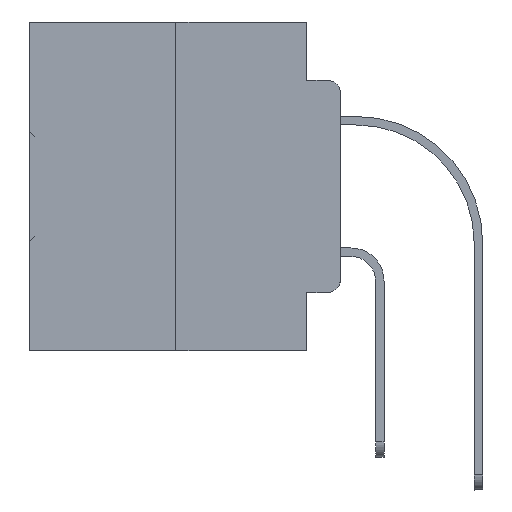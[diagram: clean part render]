
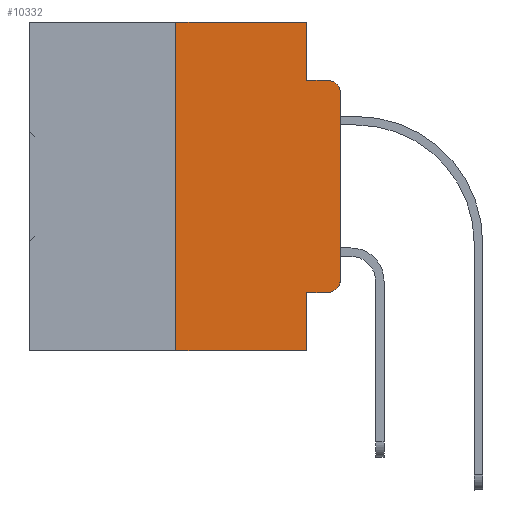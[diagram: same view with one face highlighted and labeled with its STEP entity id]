
A CAD part, left-side view. The second image highlights one B-rep face of the part: STEP entity #10332.
In plain terms, the highlighted planar face has unit normal (-1, 0, 0).
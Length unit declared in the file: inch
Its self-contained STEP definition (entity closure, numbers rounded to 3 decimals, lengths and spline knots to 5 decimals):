
#187 = ORIENTED_EDGE ( 'NONE', *, *, #8697, .T. ) ;
#193 = ORIENTED_EDGE ( 'NONE', *, *, #16590, .F. ) ;
#374 = CARTESIAN_POINT ( 'NONE',  ( 0., 0.051, 0. ) ) ;
#519 = EDGE_CURVE ( 'NONE', #16390, #2244, #39114, .T. ) ;
#630 = CARTESIAN_POINT ( 'NONE',  ( 0., 0.051, 0. ) ) ;
#1103 = ORIENTED_EDGE ( 'NONE', *, *, #519, .T. ) ;
#1309 = EDGE_LOOP ( 'NONE', ( #1103, #26729, #22844, #6492, #193, #5804, #22994, #35599, #187, #27487 ) ) ;
#1374 = DIRECTION ( 'NONE',  ( -1., 0., 0. ) ) ;
#1919 = CARTESIAN_POINT ( 'NONE',  ( 0., 0.051, 0. ) ) ;
#2244 = VERTEX_POINT ( 'NONE', #14629 ) ;
#3180 = VECTOR ( 'NONE', #23820, 39.37008 ) ;
#3497 = EDGE_CURVE ( 'NONE', #2244, #32192, #19511, .T. ) ;
#3555 = DIRECTION ( 'NONE',  ( 0., 0., -1. ) ) ;
#3801 = CARTESIAN_POINT ( 'NONE',  ( 0., 0.051, -0.0885 ) ) ;
#3880 = CARTESIAN_POINT ( 'NONE',  ( 0., 0.051, -0.4115 ) ) ;
#4051 = VECTOR ( 'NONE', #3555, 39.37008 ) ;
#5753 = LINE ( 'NONE', #30187, #23988 ) ;
#5804 = ORIENTED_EDGE ( 'NONE', *, *, #35018, .F. ) ;
#6402 = PLANE ( 'NONE',  #11714 ) ;
#6492 = ORIENTED_EDGE ( 'NONE', *, *, #27255, .F. ) ;
#6831 = LINE ( 'NONE', #3880, #28405 ) ;
#6949 = DIRECTION ( 'NONE',  ( 0., -1., 0. ) ) ;
#7111 = CARTESIAN_POINT ( 'NONE',  ( 0., 0.02, -0.0885 ) ) ;
#8697 = EDGE_CURVE ( 'NONE', #21291, #14840, #6831, .T. ) ;
#9057 = CARTESIAN_POINT ( 'NONE',  ( 0., 0.25, 0. ) ) ;
#10332 = ADVANCED_FACE ( 'NONE', ( #24301 ), #6402, .F. ) ;
#10700 = CARTESIAN_POINT ( 'NONE',  ( 0., 0.02, -0.1085 ) ) ;
#11714 = AXIS2_PLACEMENT_3D ( 'NONE', #30457, #32834, #30258 ) ;
#12043 = LINE ( 'NONE', #9057, #22692 ) ;
#12808 = DIRECTION ( 'NONE',  ( 0., -1., 0. ) ) ;
#12985 = CARTESIAN_POINT ( 'NONE',  ( 0., 0.051, -0.4115 ) ) ;
#13121 = CARTESIAN_POINT ( 'NONE',  ( 0., 0.051, -0.5 ) ) ;
#13343 = CARTESIAN_POINT ( 'NONE',  ( 0., 0.25, 0. ) ) ;
#14063 = DIRECTION ( 'NONE',  ( 0., 0., -1. ) ) ;
#14528 = LINE ( 'NONE', #3801, #15009 ) ;
#14554 = CARTESIAN_POINT ( 'NONE',  ( 0., 0.051, -0.0885 ) ) ;
#14629 = CARTESIAN_POINT ( 'NONE',  ( 0., 0., -0.1085 ) ) ;
#14840 = VERTEX_POINT ( 'NONE', #20939 ) ;
#15009 = VECTOR ( 'NONE', #6949, 39.37008 ) ;
#15873 = CARTESIAN_POINT ( 'NONE',  ( 0., 0.473, -0.5 ) ) ;
#16047 = VERTEX_POINT ( 'NONE', #13343 ) ;
#16390 = VERTEX_POINT ( 'NONE', #34378 ) ;
#16452 = LINE ( 'NONE', #15873, #38403 ) ;
#16590 = EDGE_CURVE ( 'NONE', #16047, #26846, #5753, .T. ) ;
#16953 = EDGE_CURVE ( 'NONE', #14840, #16390, #18135, .T. ) ;
#18135 = CIRCLE ( 'NONE', #28932, 0.02 ) ;
#19195 = CARTESIAN_POINT ( 'NONE',  ( 0., 0.25, -0.5 ) ) ;
#19511 = CIRCLE ( 'NONE', #34089, 0.02 ) ;
#19806 = VERTEX_POINT ( 'NONE', #19195 ) ;
#20008 = EDGE_CURVE ( 'NONE', #21291, #28140, #28558, .T. ) ;
#20939 = CARTESIAN_POINT ( 'NONE',  ( 0., 0.02, -0.4115 ) ) ;
#21291 = VERTEX_POINT ( 'NONE', #12985 ) ;
#22692 = VECTOR ( 'NONE', #24563, 39.37008 ) ;
#22823 = DIRECTION ( 'NONE',  ( -1., 0., 0. ) ) ;
#22844 = ORIENTED_EDGE ( 'NONE', *, *, #34128, .F. ) ;
#22994 = ORIENTED_EDGE ( 'NONE', *, *, #31013, .T. ) ;
#23820 = DIRECTION ( 'NONE',  ( 0., 0., 1. ) ) ;
#23988 = VECTOR ( 'NONE', #35759, 39.37008 ) ;
#24301 = FACE_OUTER_BOUND ( 'NONE', #1309, .T. ) ;
#24349 = VERTEX_POINT ( 'NONE', #14554 ) ;
#24563 = DIRECTION ( 'NONE',  ( 0., 0., 1. ) ) ;
#25266 = VECTOR ( 'NONE', #32108, 39.37008 ) ;
#26729 = ORIENTED_EDGE ( 'NONE', *, *, #3497, .T. ) ;
#26846 = VERTEX_POINT ( 'NONE', #630 ) ;
#27255 = EDGE_CURVE ( 'NONE', #26846, #24349, #36338, .T. ) ;
#27487 = ORIENTED_EDGE ( 'NONE', *, *, #16953, .T. ) ;
#28014 = DIRECTION ( 'NONE',  ( 0., -1., 0. ) ) ;
#28140 = VERTEX_POINT ( 'NONE', #13121 ) ;
#28405 = VECTOR ( 'NONE', #12808, 39.37008 ) ;
#28558 = LINE ( 'NONE', #1919, #25266 ) ;
#28932 = AXIS2_PLACEMENT_3D ( 'NONE', #31945, #1374, #14063 ) ;
#30187 = CARTESIAN_POINT ( 'NONE',  ( 0., 0.473, 0. ) ) ;
#30258 = DIRECTION ( 'NONE',  ( 0., 0., -1. ) ) ;
#30457 = CARTESIAN_POINT ( 'NONE',  ( 0., 0.473, 0. ) ) ;
#31013 = EDGE_CURVE ( 'NONE', #19806, #28140, #16452, .T. ) ;
#31748 = DIRECTION ( 'NONE',  ( 0., 0., -1. ) ) ;
#31945 = CARTESIAN_POINT ( 'NONE',  ( 0., 0.02, -0.3915 ) ) ;
#32108 = DIRECTION ( 'NONE',  ( 0., 0., -1. ) ) ;
#32192 = VERTEX_POINT ( 'NONE', #7111 ) ;
#32368 = CARTESIAN_POINT ( 'NONE',  ( 0., 0., 0. ) ) ;
#32834 = DIRECTION ( 'NONE',  ( 1., 0., 0. ) ) ;
#34089 = AXIS2_PLACEMENT_3D ( 'NONE', #10700, #22823, #31748 ) ;
#34128 = EDGE_CURVE ( 'NONE', #24349, #32192, #14528, .T. ) ;
#34378 = CARTESIAN_POINT ( 'NONE',  ( 0., 0., -0.3915 ) ) ;
#35018 = EDGE_CURVE ( 'NONE', #19806, #16047, #12043, .T. ) ;
#35599 = ORIENTED_EDGE ( 'NONE', *, *, #20008, .F. ) ;
#35759 = DIRECTION ( 'NONE',  ( 0., -1., 0. ) ) ;
#36338 = LINE ( 'NONE', #374, #4051 ) ;
#38403 = VECTOR ( 'NONE', #28014, 39.37008 ) ;
#39114 = LINE ( 'NONE', #32368, #3180 ) ;
